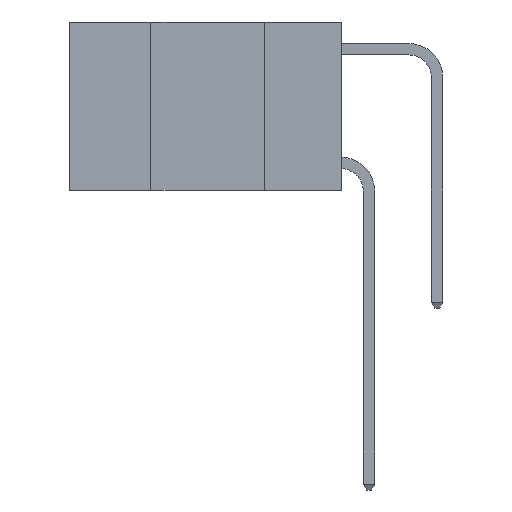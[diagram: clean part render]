
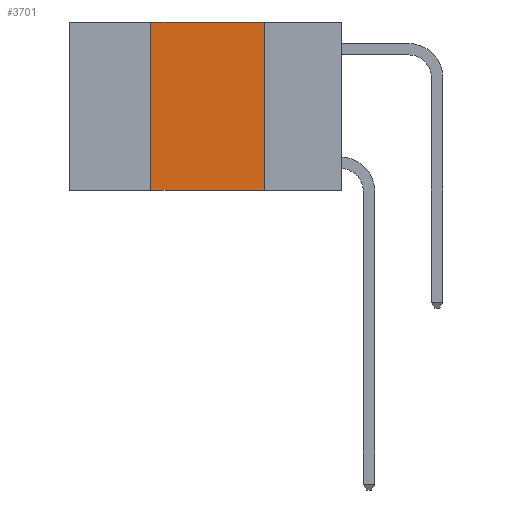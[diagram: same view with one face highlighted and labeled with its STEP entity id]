
A CAD part, left-side view. The second image highlights one B-rep face of the part: STEP entity #3701.
In plain terms, the highlighted planar face has unit normal (-1, 0, 0).
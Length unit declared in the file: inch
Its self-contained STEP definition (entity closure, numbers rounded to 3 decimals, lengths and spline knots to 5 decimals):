
#10 = VERTEX_POINT ( 'NONE', #4926 ) ;
#304 = CARTESIAN_POINT ( 'NONE',  ( 0., 0.42, -0.37 ) ) ;
#461 = DIRECTION ( 'NONE',  ( 0., 0., -1. ) ) ;
#533 = CARTESIAN_POINT ( 'NONE',  ( 0., 0.17, 0. ) ) ;
#576 = LINE ( 'NONE', #1986, #8339 ) ;
#596 = EDGE_LOOP ( 'NONE', ( #3433, #3494, #3563, #3629 ) ) ;
#1017 = LINE ( 'NONE', #10185, #5900 ) ;
#1449 = CARTESIAN_POINT ( 'NONE',  ( 0., 0.17, 0. ) ) ;
#1555 = DIRECTION ( 'NONE',  ( 0., -1., 0. ) ) ;
#1986 = CARTESIAN_POINT ( 'NONE',  ( 0., 0.6, -0.37 ) ) ;
#2700 = AXIS2_PLACEMENT_3D ( 'NONE', #10812, #11750, #6049 ) ;
#2776 = VERTEX_POINT ( 'NONE', #1449 ) ;
#2879 = EDGE_CURVE ( 'NONE', #2776, #10, #10245, .T. ) ;
#2967 = DIRECTION ( 'NONE',  ( 0., -1., 0. ) ) ;
#3433 = ORIENTED_EDGE ( 'NONE', *, *, #2879, .F. ) ;
#3494 = ORIENTED_EDGE ( 'NONE', *, *, #10672, .F. ) ;
#3563 = ORIENTED_EDGE ( 'NONE', *, *, #8771, .F. ) ;
#3629 = ORIENTED_EDGE ( 'NONE', *, *, #9645, .T. ) ;
#3701 = ADVANCED_FACE ( 'NONE', ( #8290 ), #4118, .F. ) ;
#4118 = PLANE ( 'NONE',  #2700 ) ;
#4450 = VERTEX_POINT ( 'NONE', #304 ) ;
#4835 = CARTESIAN_POINT ( 'NONE',  ( 0., 0.42, 0. ) ) ;
#4926 = CARTESIAN_POINT ( 'NONE',  ( 0., 0.17, -0.37 ) ) ;
#5210 = LINE ( 'NONE', #9379, #7448 ) ;
#5900 = VECTOR ( 'NONE', #1555, 39.37008 ) ;
#6049 = DIRECTION ( 'NONE',  ( 0., 0., -1. ) ) ;
#7448 = VECTOR ( 'NONE', #12205, 39.37008 ) ;
#7709 = VECTOR ( 'NONE', #461, 39.37008 ) ;
#8290 = FACE_OUTER_BOUND ( 'NONE', #596, .T. ) ;
#8339 = VECTOR ( 'NONE', #2967, 39.37008 ) ;
#8771 = EDGE_CURVE ( 'NONE', #4450, #10911, #5210, .T. ) ;
#9379 = CARTESIAN_POINT ( 'NONE',  ( 0., 0.42, 0. ) ) ;
#9645 = EDGE_CURVE ( 'NONE', #4450, #10, #576, .T. ) ;
#10185 = CARTESIAN_POINT ( 'NONE',  ( 0., 0.6, 0. ) ) ;
#10245 = LINE ( 'NONE', #533, #7709 ) ;
#10672 = EDGE_CURVE ( 'NONE', #10911, #2776, #1017, .T. ) ;
#10812 = CARTESIAN_POINT ( 'NONE',  ( 0., 0.6, 0. ) ) ;
#10911 = VERTEX_POINT ( 'NONE', #4835 ) ;
#11750 = DIRECTION ( 'NONE',  ( 1., 0., 0. ) ) ;
#12205 = DIRECTION ( 'NONE',  ( 0., 0., 1. ) ) ;
